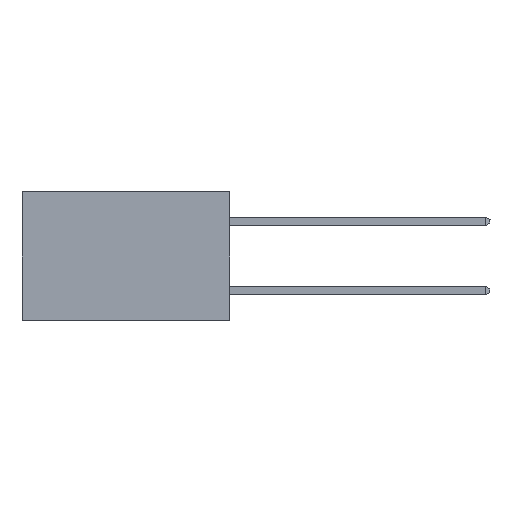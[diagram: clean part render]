
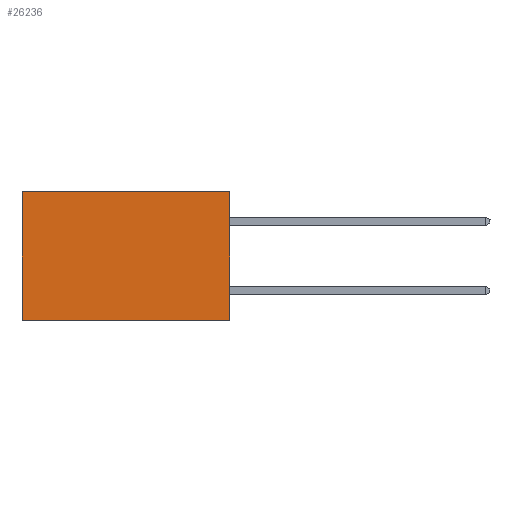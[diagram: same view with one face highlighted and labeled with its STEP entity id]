
A CAD part, left-side view. The second image highlights one B-rep face of the part: STEP entity #26236.
In plain terms, the highlighted planar face has unit normal (-1, 0, 0).
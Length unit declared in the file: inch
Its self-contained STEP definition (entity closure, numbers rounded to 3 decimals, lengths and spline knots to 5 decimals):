
#170 = ORIENTED_EDGE ( 'NONE', *, *, #5076, .F. ) ;
#320 = CARTESIAN_POINT ( 'NONE',  ( 0.2615, 0., -0.37 ) ) ;
#924 = EDGE_CURVE ( 'NONE', #17753, #3930, #7721, .T. ) ;
#1283 = VERTEX_POINT ( 'NONE', #8923 ) ;
#1467 = CARTESIAN_POINT ( 'NONE',  ( 0.2615, 0., 0. ) ) ;
#1860 = DIRECTION ( 'NONE',  ( 0., 1., 0. ) ) ;
#2560 = ORIENTED_EDGE ( 'NONE', *, *, #9516, .T. ) ;
#3053 = VECTOR ( 'NONE', #24151, 39.37008 ) ;
#3930 = VERTEX_POINT ( 'NONE', #320 ) ;
#4431 = FACE_OUTER_BOUND ( 'NONE', #26393, .T. ) ;
#5076 = EDGE_CURVE ( 'NONE', #3930, #1283, #8330, .T. ) ;
#5547 = DIRECTION ( 'NONE',  ( 0., 0., -1. ) ) ;
#5568 = VECTOR ( 'NONE', #20643, 39.37008 ) ;
#7206 = ORIENTED_EDGE ( 'NONE', *, *, #16195, .T. ) ;
#7295 = CARTESIAN_POINT ( 'NONE',  ( 0.2615, 0.6, -0.37 ) ) ;
#7721 = LINE ( 'NONE', #19955, #3053 ) ;
#8222 = ORIENTED_EDGE ( 'NONE', *, *, #924, .F. ) ;
#8330 = LINE ( 'NONE', #22850, #12362 ) ;
#8399 = CARTESIAN_POINT ( 'NONE',  ( 0.2615, 0., 0. ) ) ;
#8923 = CARTESIAN_POINT ( 'NONE',  ( 0.2615, 0.6, -0.37 ) ) ;
#9516 = EDGE_CURVE ( 'NONE', #17753, #17079, #18993, .T. ) ;
#11322 = CARTESIAN_POINT ( 'NONE',  ( 0.2615, 0.6, 0. ) ) ;
#12362 = VECTOR ( 'NONE', #1860, 39.37008 ) ;
#14645 = AXIS2_PLACEMENT_3D ( 'NONE', #25200, #20997, #14748 ) ;
#14748 = DIRECTION ( 'NONE',  ( 0., 0., -1. ) ) ;
#14881 = PLANE ( 'NONE',  #14645 ) ;
#16195 = EDGE_CURVE ( 'NONE', #17079, #1283, #23863, .T. ) ;
#17008 = VECTOR ( 'NONE', #5547, 39.37008 ) ;
#17079 = VERTEX_POINT ( 'NONE', #11322 ) ;
#17753 = VERTEX_POINT ( 'NONE', #1467 ) ;
#18993 = LINE ( 'NONE', #8399, #5568 ) ;
#19955 = CARTESIAN_POINT ( 'NONE',  ( 0.2615, 0., -0.37 ) ) ;
#20643 = DIRECTION ( 'NONE',  ( 0., 1., 0. ) ) ;
#20997 = DIRECTION ( 'NONE',  ( 1., 0., 0. ) ) ;
#22850 = CARTESIAN_POINT ( 'NONE',  ( 0.2615, 0., -0.37 ) ) ;
#23863 = LINE ( 'NONE', #7295, #17008 ) ;
#24151 = DIRECTION ( 'NONE',  ( 0., 0., -1. ) ) ;
#25200 = CARTESIAN_POINT ( 'NONE',  ( 0.2615, 0., -0.37 ) ) ;
#26236 = ADVANCED_FACE ( 'NONE', ( #4431 ), #14881, .F. ) ;
#26393 = EDGE_LOOP ( 'NONE', ( #7206, #170, #8222, #2560 ) ) ;
